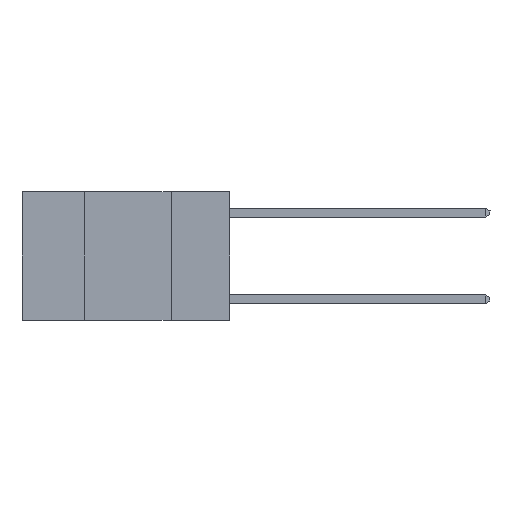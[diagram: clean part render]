
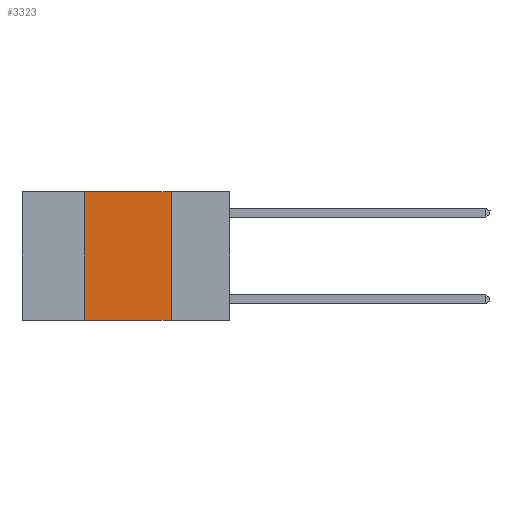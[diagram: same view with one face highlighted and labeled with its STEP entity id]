
A CAD part, left-side view. The second image highlights one B-rep face of the part: STEP entity #3323.
In plain terms, the highlighted planar face has unit normal (-1, 0, 0).
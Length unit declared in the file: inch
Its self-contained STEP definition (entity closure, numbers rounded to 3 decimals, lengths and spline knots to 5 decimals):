
#20 = AXIS2_PLACEMENT_3D ( 'NONE', #66, #6271, #5603 ) ;
#66 = CARTESIAN_POINT ( 'NONE',  ( 0., 0.6, 0. ) ) ;
#93 = LINE ( 'NONE', #1838, #2136 ) ;
#1053 = EDGE_CURVE ( 'NONE', #9032, #10731, #93, .T. ) ;
#1055 = CARTESIAN_POINT ( 'NONE',  ( 0., 0.6, -0.37 ) ) ;
#1818 = VERTEX_POINT ( 'NONE', #3793 ) ;
#1838 = CARTESIAN_POINT ( 'NONE',  ( 0., 0.6, 0. ) ) ;
#1961 = DIRECTION ( 'NONE',  ( 0., 0., 1. ) ) ;
#2136 = VECTOR ( 'NONE', #8629, 39.37008 ) ;
#2501 = LINE ( 'NONE', #8172, #6774 ) ;
#3323 = ADVANCED_FACE ( 'NONE', ( #8852 ), #4514, .F. ) ;
#3692 = CARTESIAN_POINT ( 'NONE',  ( 0., 0.42, 0. ) ) ;
#3793 = CARTESIAN_POINT ( 'NONE',  ( 0., 0.17, -0.37 ) ) ;
#3923 = VERTEX_POINT ( 'NONE', #10341 ) ;
#4514 = PLANE ( 'NONE',  #20 ) ;
#4548 = LINE ( 'NONE', #1055, #5978 ) ;
#4720 = EDGE_CURVE ( 'NONE', #10731, #1818, #2501, .T. ) ;
#4819 = ORIENTED_EDGE ( 'NONE', *, *, #4720, .F. ) ;
#5281 = ORIENTED_EDGE ( 'NONE', *, *, #10063, .F. ) ;
#5603 = DIRECTION ( 'NONE',  ( 0., 0., -1. ) ) ;
#5978 = VECTOR ( 'NONE', #7005, 39.37008 ) ;
#6266 = LINE ( 'NONE', #3692, #8497 ) ;
#6271 = DIRECTION ( 'NONE',  ( 1., 0., 0. ) ) ;
#6774 = VECTOR ( 'NONE', #9025, 39.37008 ) ;
#7005 = DIRECTION ( 'NONE',  ( 0., -1., 0. ) ) ;
#7099 = CARTESIAN_POINT ( 'NONE',  ( 0., 0.17, 0. ) ) ;
#7358 = CARTESIAN_POINT ( 'NONE',  ( 0., 0.42, 0. ) ) ;
#7995 = ORIENTED_EDGE ( 'NONE', *, *, #8729, .T. ) ;
#8172 = CARTESIAN_POINT ( 'NONE',  ( 0., 0.17, 0. ) ) ;
#8497 = VECTOR ( 'NONE', #1961, 39.37008 ) ;
#8629 = DIRECTION ( 'NONE',  ( 0., -1., 0. ) ) ;
#8729 = EDGE_CURVE ( 'NONE', #3923, #1818, #4548, .T. ) ;
#8852 = FACE_OUTER_BOUND ( 'NONE', #10020, .T. ) ;
#9025 = DIRECTION ( 'NONE',  ( 0., 0., -1. ) ) ;
#9032 = VERTEX_POINT ( 'NONE', #7358 ) ;
#9184 = ORIENTED_EDGE ( 'NONE', *, *, #1053, .F. ) ;
#10020 = EDGE_LOOP ( 'NONE', ( #4819, #9184, #5281, #7995 ) ) ;
#10063 = EDGE_CURVE ( 'NONE', #3923, #9032, #6266, .T. ) ;
#10341 = CARTESIAN_POINT ( 'NONE',  ( 0., 0.42, -0.37 ) ) ;
#10731 = VERTEX_POINT ( 'NONE', #7099 ) ;
